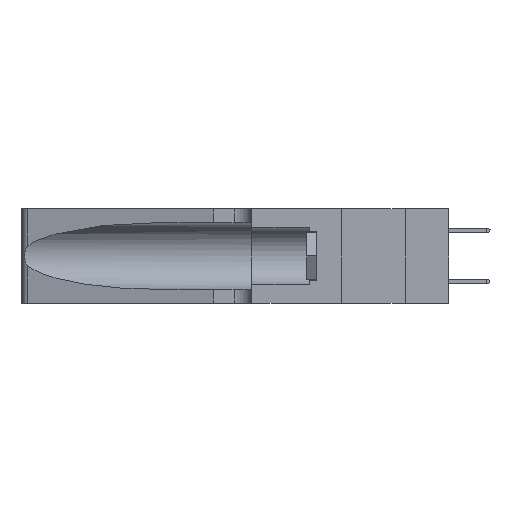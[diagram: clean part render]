
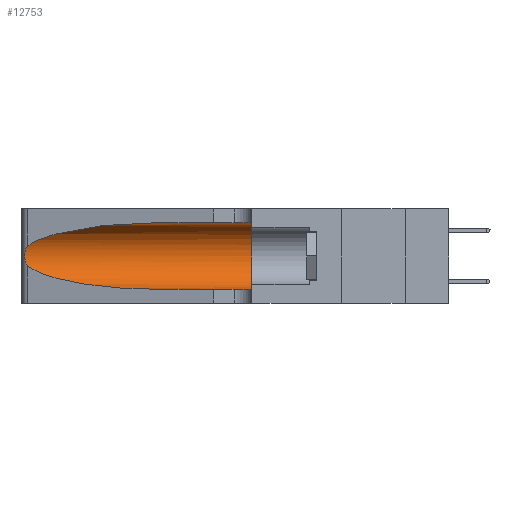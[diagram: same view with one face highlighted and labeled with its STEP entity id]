
A CAD part, left-side view. The second image highlights one B-rep face of the part: STEP entity #12753.
In plain terms, the highlighted cylindrical face has radius 3.308 mm (diameter 6.617 mm), a partial arc.
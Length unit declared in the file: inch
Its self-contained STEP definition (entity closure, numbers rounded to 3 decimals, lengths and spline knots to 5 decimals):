
#103 = CARTESIAN_POINT ( 'NONE',  ( 0.26075, 1.23896, 0.19203 ) ) ;
#448 = CARTESIAN_POINT ( 'NONE',  ( 0.1305, 0.35, 0.05475 ) ) ;
#1028 = VERTEX_POINT ( 'NONE', #18416 ) ;
#1038 = CARTESIAN_POINT ( 'NONE',  ( 0.2373, 1.15595, 0.08982 ) ) ;
#2335 = FACE_OUTER_BOUND ( 'NONE', #14595, .T. ) ;
#2506 = CARTESIAN_POINT ( 'NONE',  ( 0.1305, 0.72297, 0.05475 ) ) ;
#3028 = CYLINDRICAL_SURFACE ( 'NONE', #10503, 0.13025 ) ;
#3516 = AXIS2_PLACEMENT_3D ( 'NONE', #17395, #10027, #5626 ) ;
#3863 = CARTESIAN_POINT ( 'NONE',  ( 0.18966, 0.96281, 0.05475 ) ) ;
#4030 = CARTESIAN_POINT ( 'NONE',  ( 0.25487, 1.22718, 0.14631 ) ) ;
#4190 = ORIENTED_EDGE ( 'NONE', *, *, #18437, .F. ) ;
#4542 = CARTESIAN_POINT ( 'NONE',  ( 0.25555, 1.22993, 0.14849 ) ) ;
#4602 = CARTESIAN_POINT ( 'NONE',  ( 0.26018, 1.23835, 0.19895 ) ) ;
#4745 = EDGE_CURVE ( 'NONE', #13142, #14694, #10700, .T. ) ;
#5311 = EDGE_CURVE ( 'NONE', #1028, #9347, #5719, .T. ) ;
#5375 = ORIENTED_EDGE ( 'NONE', *, *, #9696, .T. ) ;
#5626 = DIRECTION ( 'NONE',  ( 0., 0., 1. ) ) ;
#5719 = B_SPLINE_CURVE_WITH_KNOTS ( 'NONE', 3,
 ( #14806, #16298, #8039, #17771, #8856, #4602, #103, #14999, #6134, #10403, #10277, #14746, #4542, #17838 ),
 .UNSPECIFIED., .F., .F.,
 ( 4, 2, 2, 2, 2, 2, 4 ),
 ( 0., 0.00027, 0.00053, 0.00107, 0.0016, 0.00187, 0.00214 ),
 .UNSPECIFIED. ) ;
#6134 = CARTESIAN_POINT ( 'NONE',  ( 0.26017, 1.23833, 0.17102 ) ) ;
#6312 = ORIENTED_EDGE ( 'NONE', *, *, #7391, .T. ) ;
#6644 = DIRECTION ( 'NONE',  ( 0., 0., -1. ) ) ;
#6756 = DIRECTION ( 'NONE',  ( 0., -1., 0. ) ) ;
#7361 = CARTESIAN_POINT ( 'NONE',  ( 0.1305, 0.35, 0.31525 ) ) ;
#7391 = EDGE_CURVE ( 'NONE', #13603, #14694, #7682, .T. ) ;
#7682 = LINE ( 'NONE', #18359, #10248 ) ;
#8039 = CARTESIAN_POINT ( 'NONE',  ( 0.25639, 1.23184, 0.21858 ) ) ;
#8856 = CARTESIAN_POINT ( 'NONE',  ( 0.25854, 1.2359, 0.20912 ) ) ;
#9347 = VERTEX_POINT ( 'NONE', #4030 ) ;
#9696 = EDGE_CURVE ( 'NONE', #15232, #1028, #14380, .T. ) ;
#9823 = CARTESIAN_POINT ( 'NONE',  ( 0.18966, 0.96281, 0.31525 ) ) ;
#10027 = DIRECTION ( 'NONE',  ( 0., 1., 0. ) ) ;
#10248 = VECTOR ( 'NONE', #17072, 39.37008 ) ;
#10277 = CARTESIAN_POINT ( 'NONE',  ( 0.25789, 1.23486, 0.15765 ) ) ;
#10403 = CARTESIAN_POINT ( 'NONE',  ( 0.25856, 1.23593, 0.16098 ) ) ;
#10503 = AXIS2_PLACEMENT_3D ( 'NONE', #11348, #6756, #6644 ) ;
#10700 = CIRCLE ( 'NONE', #3516, 0.13025 ) ;
#10823 = CARTESIAN_POINT ( 'NONE',  ( 0.25487, 1.22718, 0.14631 ) ) ;
#11348 = CARTESIAN_POINT ( 'NONE',  ( 0.1305, 1.61858, 0.185 ) ) ;
#11392 = CARTESIAN_POINT ( 'NONE',  ( 0.1305, 1.61858, 0.31525 ) ) ;
#11487 = ORIENTED_EDGE ( 'NONE', *, *, #5311, .T. ) ;
#11842 = VECTOR ( 'NONE', #15708, 39.37008 ) ;
#12146 = CARTESIAN_POINT ( 'NONE',  ( 0.25487, 1.22718, 0.22369 ) ) ;
#12753 = ADVANCED_FACE ( 'NONE', ( #2335 ), #3028, .F. ) ;
#12857 = CARTESIAN_POINT ( 'NONE',  ( 0.1305, 0.72297, 0.31525 ) ) ;
#13142 = VERTEX_POINT ( 'NONE', #7361 ) ;
#13475 = CARTESIAN_POINT ( 'NONE',  ( 0.1305, 0.72297, 0.05475 ) ) ;
#13603 = VERTEX_POINT ( 'NONE', #13475 ) ;
#14343 = EDGE_CURVE ( 'NONE', #9347, #13603, #18396, .T. ) ;
#14380 =( BOUNDED_CURVE ( )  B_SPLINE_CURVE ( 3, ( #15650, #9823, #16417, #12146 ),
 .UNSPECIFIED., .F., .F. ) 
 B_SPLINE_CURVE_WITH_KNOTS ( ( 4, 4 ),
 ( 1.5708, 2.84003 ),
 .UNSPECIFIED. ) 
 CURVE ( )  GEOMETRIC_REPRESENTATION_ITEM ( )  RATIONAL_B_SPLINE_CURVE ( ( 1., 0.87, 0.87, 1. ) ) 
 REPRESENTATION_ITEM ( '' )  );
#14595 = EDGE_LOOP ( 'NONE', ( #5375, #11487, #17493, #6312, #18284, #4190 ) ) ;
#14694 = VERTEX_POINT ( 'NONE', #448 ) ;
#14746 = CARTESIAN_POINT ( 'NONE',  ( 0.25639, 1.23186, 0.15144 ) ) ;
#14806 = CARTESIAN_POINT ( 'NONE',  ( 0.25487, 1.22718, 0.22369 ) ) ;
#14999 = CARTESIAN_POINT ( 'NONE',  ( 0.26075, 1.23896, 0.178 ) ) ;
#15232 = VERTEX_POINT ( 'NONE', #12857 ) ;
#15650 = CARTESIAN_POINT ( 'NONE',  ( 0.1305, 0.72297, 0.31525 ) ) ;
#15708 = DIRECTION ( 'NONE',  ( 0., -1., 0. ) ) ;
#15766 = LINE ( 'NONE', #11392, #11842 ) ;
#16298 = CARTESIAN_POINT ( 'NONE',  ( 0.25555, 1.22994, 0.2215 ) ) ;
#16417 = CARTESIAN_POINT ( 'NONE',  ( 0.2373, 1.15595, 0.28018 ) ) ;
#17072 = DIRECTION ( 'NONE',  ( 0., -1., 0. ) ) ;
#17395 = CARTESIAN_POINT ( 'NONE',  ( 0.1305, 0.35, 0.185 ) ) ;
#17493 = ORIENTED_EDGE ( 'NONE', *, *, #14343, .T. ) ;
#17771 = CARTESIAN_POINT ( 'NONE',  ( 0.25787, 1.23484, 0.2124 ) ) ;
#17838 = CARTESIAN_POINT ( 'NONE',  ( 0.25487, 1.22718, 0.14631 ) ) ;
#18284 = ORIENTED_EDGE ( 'NONE', *, *, #4745, .F. ) ;
#18359 = CARTESIAN_POINT ( 'NONE',  ( 0.1305, 1.61858, 0.05475 ) ) ;
#18396 =( BOUNDED_CURVE ( )  B_SPLINE_CURVE ( 3, ( #10823, #1038, #3863, #2506 ),
 .UNSPECIFIED., .F., .T. ) 
 B_SPLINE_CURVE_WITH_KNOTS ( ( 4, 4 ),
 ( 3.44316, 4.71239 ),
 .UNSPECIFIED. ) 
 CURVE ( )  GEOMETRIC_REPRESENTATION_ITEM ( )  RATIONAL_B_SPLINE_CURVE ( ( 1., 0.87, 0.87, 1. ) ) 
 REPRESENTATION_ITEM ( '' )  );
#18416 = CARTESIAN_POINT ( 'NONE',  ( 0.25487, 1.22718, 0.22369 ) ) ;
#18437 = EDGE_CURVE ( 'NONE', #15232, #13142, #15766, .T. ) ;
